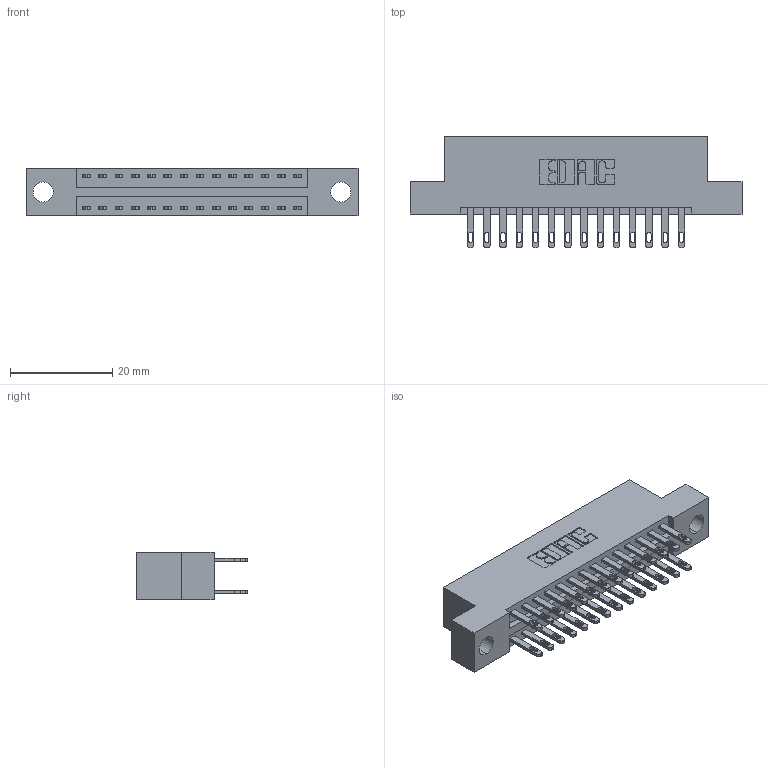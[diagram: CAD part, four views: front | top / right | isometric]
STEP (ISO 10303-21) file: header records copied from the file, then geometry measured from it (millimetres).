
FILE_DESCRIPTION (( 'STEP AP203' ), '1' );
FILE_NAME ('346-028-500-204.STEP', '2018-08-22T00:40:38', ( '' ), ( '' ), 'SwSTEP 2.0', 'SolidWorks 2016', '' );
FILE_SCHEMA (( 'CONFIG_CONTROL_DESIGN' ));
Length unit declared in the file: inch
Products named in the file (3): 346 Part_Flush Mounting Lugs - 0.156 Dia-TH; 345-292-001_345-293-100; 346-028-500-204
Assembly tree (29 placements, depth 2):
  346-028-500-204
    346 Part_Flush Mounting Lugs - 0.156 Dia-TH
    345-292-001_345-293-100  x28
Bounding box: 65.02 x 21.84 x 9.4 mm (x, y, z)
Volume: 6120.9 mm3; surface area: 8079.9 mm2
Topology: 29 solids, 29 shells, 1466 faces, 4445 edges, 2962 vertices
Faces by surface type: plane 888, cylinder 578
Entity records: 12839 total; most frequent: CARTESIAN_POINT 2152, ORIENTED_EDGE 2086, DIRECTION 1951, EDGE_CURVE 1043, LINE 851, VECTOR 851, VERTEX_POINT 694, AXIS2_PLACEMENT_3D 550
